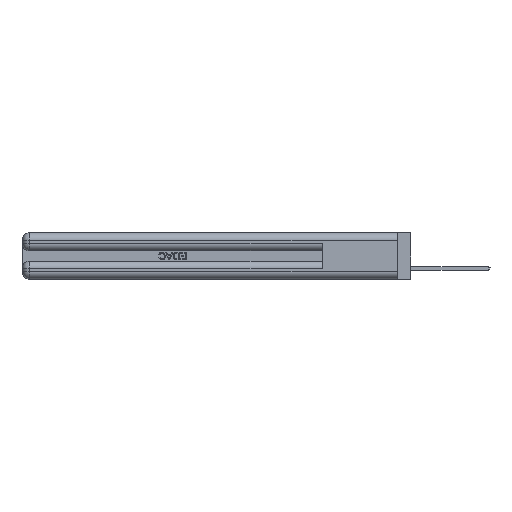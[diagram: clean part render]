
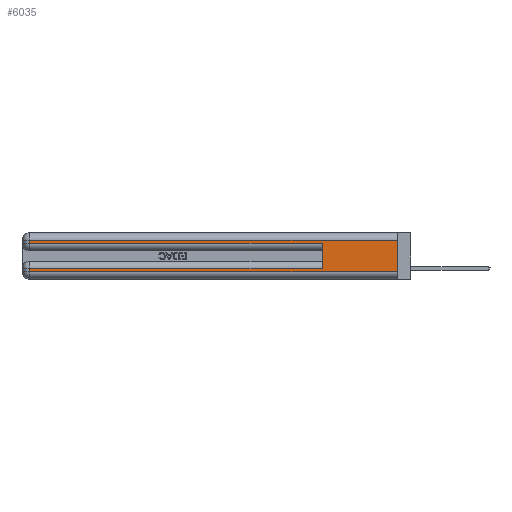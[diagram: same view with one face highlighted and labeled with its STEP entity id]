
A CAD part, left-side view. The second image highlights one B-rep face of the part: STEP entity #6035.
In plain terms, the highlighted planar face has unit normal (-1, 0, 0).
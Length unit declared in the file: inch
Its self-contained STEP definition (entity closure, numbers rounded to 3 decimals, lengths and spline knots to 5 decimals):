
#183 = ORIENTED_EDGE ( 'NONE', *, *, #5402, .F. ) ;
#257 = VERTEX_POINT ( 'NONE', #23593 ) ;
#658 = VERTEX_POINT ( 'NONE', #17884 ) ;
#1179 = VERTEX_POINT ( 'NONE', #15712 ) ;
#1712 = VERTEX_POINT ( 'NONE', #23711 ) ;
#2128 = FACE_OUTER_BOUND ( 'NONE', #7177, .T. ) ;
#3224 = VECTOR ( 'NONE', #7286, 39.37008 ) ;
#3253 = DIRECTION ( 'NONE',  ( 1., 0., 0. ) ) ;
#5402 = EDGE_CURVE ( 'NONE', #257, #658, #11845, .T. ) ;
#6035 = ADVANCED_FACE ( 'NONE', ( #2128 ), #42580, .F. ) ;
#6843 = CARTESIAN_POINT ( 'NONE',  ( 0., 2.94, 0.285 ) ) ;
#7177 = EDGE_LOOP ( 'NONE', ( #32067, #33483, #25183, #12955, #183, #13608, #38322, #11255 ) ) ;
#7286 = DIRECTION ( 'NONE',  ( 0., 0., -1. ) ) ;
#7420 = CARTESIAN_POINT ( 'NONE',  ( 0., 0., 0.37 ) ) ;
#8624 = EDGE_CURVE ( 'NONE', #18998, #1712, #16205, .T. ) ;
#10766 = VECTOR ( 'NONE', #13419, 39.37008 ) ;
#11255 = ORIENTED_EDGE ( 'NONE', *, *, #31628, .T. ) ;
#11770 = DIRECTION ( 'NONE',  ( 0., 0., -1. ) ) ;
#11845 = LINE ( 'NONE', #29257, #15757 ) ;
#12043 = CARTESIAN_POINT ( 'NONE',  ( 0., 2.94, 0.37 ) ) ;
#12351 = CARTESIAN_POINT ( 'NONE',  ( 0., 0., 0.31 ) ) ;
#12636 = LINE ( 'NONE', #40465, #27908 ) ;
#12955 = ORIENTED_EDGE ( 'NONE', *, *, #28922, .T. ) ;
#13419 = DIRECTION ( 'NONE',  ( 0., -1., 0. ) ) ;
#13608 = ORIENTED_EDGE ( 'NONE', *, *, #25613, .T. ) ;
#14711 = VECTOR ( 'NONE', #29709, 39.37008 ) ;
#15712 = CARTESIAN_POINT ( 'NONE',  ( 0., 2.94, 0.31 ) ) ;
#15757 = VECTOR ( 'NONE', #21982, 39.37008 ) ;
#15907 = DIRECTION ( 'NONE',  ( 0., 1., 0. ) ) ;
#16205 = LINE ( 'NONE', #7420, #3224 ) ;
#16540 = CARTESIAN_POINT ( 'NONE',  ( 0., 0., 0.285 ) ) ;
#17884 = CARTESIAN_POINT ( 'NONE',  ( 0., 0.6, 0.285 ) ) ;
#18998 = VERTEX_POINT ( 'NONE', #32806 ) ;
#20141 = CARTESIAN_POINT ( 'NONE',  ( 0., 0., 0.06 ) ) ;
#20818 = VERTEX_POINT ( 'NONE', #38918 ) ;
#21593 = CARTESIAN_POINT ( 'NONE',  ( 0., 0., 0.37 ) ) ;
#21982 = DIRECTION ( 'NONE',  ( 0., 0., 1. ) ) ;
#23049 = VECTOR ( 'NONE', #33982, 39.37008 ) ;
#23593 = CARTESIAN_POINT ( 'NONE',  ( 0., 0.6, 0.085 ) ) ;
#23711 = CARTESIAN_POINT ( 'NONE',  ( 0., 0., 0.06 ) ) ;
#24030 = LINE ( 'NONE', #16540, #26223 ) ;
#25183 = ORIENTED_EDGE ( 'NONE', *, *, #29790, .T. ) ;
#25513 = LINE ( 'NONE', #12351, #43537 ) ;
#25613 = EDGE_CURVE ( 'NONE', #257, #41341, #45669, .T. ) ;
#26223 = VECTOR ( 'NONE', #32542, 39.37008 ) ;
#27908 = VECTOR ( 'NONE', #11770, 39.37008 ) ;
#28922 = EDGE_CURVE ( 'NONE', #34110, #658, #24030, .T. ) ;
#29257 = CARTESIAN_POINT ( 'NONE',  ( 0., 0.6, 0.145 ) ) ;
#29709 = DIRECTION ( 'NONE',  ( 0., 0., -1. ) ) ;
#29790 = EDGE_CURVE ( 'NONE', #1179, #34110, #12636, .T. ) ;
#31628 = EDGE_CURVE ( 'NONE', #20818, #1712, #44551, .T. ) ;
#31723 = LINE ( 'NONE', #12043, #14711 ) ;
#32067 = ORIENTED_EDGE ( 'NONE', *, *, #8624, .F. ) ;
#32542 = DIRECTION ( 'NONE',  ( 0., -1., 0. ) ) ;
#32806 = CARTESIAN_POINT ( 'NONE',  ( 0., 0., 0.31 ) ) ;
#33483 = ORIENTED_EDGE ( 'NONE', *, *, #35751, .T. ) ;
#33982 = DIRECTION ( 'NONE',  ( 0., 1., 0. ) ) ;
#34110 = VERTEX_POINT ( 'NONE', #6843 ) ;
#35751 = EDGE_CURVE ( 'NONE', #18998, #1179, #25513, .T. ) ;
#36521 = CARTESIAN_POINT ( 'NONE',  ( 0., 2.94, 0.085 ) ) ;
#37425 = CARTESIAN_POINT ( 'NONE',  ( 0., 0., 0.085 ) ) ;
#38322 = ORIENTED_EDGE ( 'NONE', *, *, #45685, .T. ) ;
#38918 = CARTESIAN_POINT ( 'NONE',  ( 0., 2.94, 0.06 ) ) ;
#39684 = AXIS2_PLACEMENT_3D ( 'NONE', #21593, #3253, #46223 ) ;
#40465 = CARTESIAN_POINT ( 'NONE',  ( 0., 2.94, 0.37 ) ) ;
#41341 = VERTEX_POINT ( 'NONE', #36521 ) ;
#42580 = PLANE ( 'NONE',  #39684 ) ;
#43537 = VECTOR ( 'NONE', #15907, 39.37008 ) ;
#44551 = LINE ( 'NONE', #20141, #10766 ) ;
#45669 = LINE ( 'NONE', #37425, #23049 ) ;
#45685 = EDGE_CURVE ( 'NONE', #41341, #20818, #31723, .T. ) ;
#46223 = DIRECTION ( 'NONE',  ( 0., 0., -1. ) ) ;
